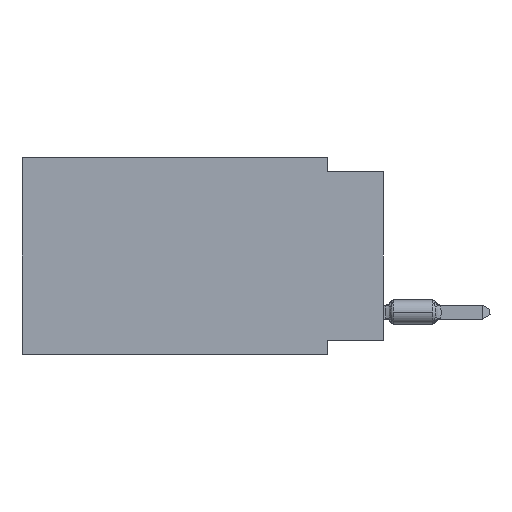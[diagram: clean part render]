
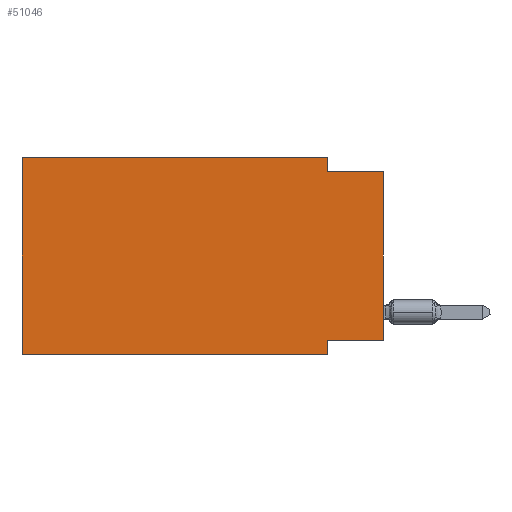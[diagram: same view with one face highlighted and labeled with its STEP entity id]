
A CAD part, left-side view. The second image highlights one B-rep face of the part: STEP entity #51046.
In plain terms, the highlighted planar face has unit normal (-1, 0, 0).
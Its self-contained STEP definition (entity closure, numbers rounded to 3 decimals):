
#1138 = ORIENTED_EDGE ( 'NONE', *, *, #31339, .F. ) ;
#1557 = VERTEX_POINT ( 'NONE', #15865 ) ;
#2071 = EDGE_CURVE ( 'NONE', #62082, #11415, #47600, .T. ) ;
#3947 = EDGE_CURVE ( 'NONE', #26505, #37810, #46423, .T. ) ;
#5848 = DIRECTION ( 'NONE',  ( 0., -1., 0. ) ) ;
#6095 = EDGE_CURVE ( 'NONE', #21302, #1557, #53220, .T. ) ;
#10886 = CARTESIAN_POINT ( 'NONE',  ( 0., 16.383, -8.89 ) ) ;
#10980 = CARTESIAN_POINT ( 'NONE',  ( 0., 16.383, 0. ) ) ;
#11415 = VERTEX_POINT ( 'NONE', #31381 ) ;
#11747 = CARTESIAN_POINT ( 'NONE',  ( 0., 0., -8.255 ) ) ;
#13044 = ORIENTED_EDGE ( 'NONE', *, *, #17821, .F. ) ;
#13174 = CARTESIAN_POINT ( 'NONE',  ( 0., 16.383, 0. ) ) ;
#14307 = ORIENTED_EDGE ( 'NONE', *, *, #48307, .T. ) ;
#15027 = CARTESIAN_POINT ( 'NONE',  ( 0., 2.54, -8.89 ) ) ;
#15865 = CARTESIAN_POINT ( 'NONE',  ( 0., 2.54, 0. ) ) ;
#16362 = PLANE ( 'NONE',  #42566 ) ;
#16434 = DIRECTION ( 'NONE',  ( 0., 1., 0. ) ) ;
#17821 = EDGE_CURVE ( 'NONE', #26505, #21302, #56416, .T. ) ;
#18202 = CARTESIAN_POINT ( 'NONE',  ( 0., 0., -8.255 ) ) ;
#19242 = LINE ( 'NONE', #28957, #56140 ) ;
#20790 = DIRECTION ( 'NONE',  ( 0., 0., 1. ) ) ;
#21302 = VERTEX_POINT ( 'NONE', #13174 ) ;
#22866 = VERTEX_POINT ( 'NONE', #36955 ) ;
#26079 = FACE_OUTER_BOUND ( 'NONE', #42232, .T. ) ;
#26472 = ORIENTED_EDGE ( 'NONE', *, *, #36853, .F. ) ;
#26487 = VECTOR ( 'NONE', #5848, 1000. ) ;
#26505 = VERTEX_POINT ( 'NONE', #48649 ) ;
#26892 = CARTESIAN_POINT ( 'NONE',  ( 0., 16.383, 0. ) ) ;
#28957 = CARTESIAN_POINT ( 'NONE',  ( 0., 0., -0.635 ) ) ;
#31339 = EDGE_CURVE ( 'NONE', #11415, #37810, #41487, .T. ) ;
#31381 = CARTESIAN_POINT ( 'NONE',  ( 0., 2.54, -8.255 ) ) ;
#31442 = DIRECTION ( 'NONE',  ( 0., 0., -1. ) ) ;
#31476 = ORIENTED_EDGE ( 'NONE', *, *, #64997, .F. ) ;
#31584 = DIRECTION ( 'NONE',  ( 0., 0., 1. ) ) ;
#31943 = VECTOR ( 'NONE', #20790, 1000. ) ;
#32130 = CARTESIAN_POINT ( 'NONE',  ( 0., 16.383, 0. ) ) ;
#36804 = DIRECTION ( 'NONE',  ( 1., 0., 0. ) ) ;
#36853 = EDGE_CURVE ( 'NONE', #1557, #38967, #57095, .T. ) ;
#36882 = VECTOR ( 'NONE', #31442, 1000. ) ;
#36955 = CARTESIAN_POINT ( 'NONE',  ( 0., 0., -0.635 ) ) ;
#37810 = VERTEX_POINT ( 'NONE', #57952 ) ;
#38967 = VERTEX_POINT ( 'NONE', #56730 ) ;
#41080 = ORIENTED_EDGE ( 'NONE', *, *, #3947, .T. ) ;
#41487 = LINE ( 'NONE', #15027, #36882 ) ;
#42232 = EDGE_LOOP ( 'NONE', ( #14307, #31476, #26472, #47606, #13044, #41080, #1138, #56118 ) ) ;
#42566 = AXIS2_PLACEMENT_3D ( 'NONE', #32130, #36804, #56618 ) ;
#46423 = LINE ( 'NONE', #10886, #26487 ) ;
#47600 = LINE ( 'NONE', #11747, #57360 ) ;
#47606 = ORIENTED_EDGE ( 'NONE', *, *, #6095, .F. ) ;
#48307 = EDGE_CURVE ( 'NONE', #62082, #22866, #61364, .T. ) ;
#48649 = CARTESIAN_POINT ( 'NONE',  ( 0., 16.383, -8.89 ) ) ;
#48747 = VECTOR ( 'NONE', #31584, 1000. ) ;
#49399 = DIRECTION ( 'NONE',  ( 0., -1., 0. ) ) ;
#51046 = ADVANCED_FACE ( 'NONE', ( #26079 ), #16362, .F. ) ;
#51198 = VECTOR ( 'NONE', #52722, 1000. ) ;
#52722 = DIRECTION ( 'NONE',  ( 0., 0., -1. ) ) ;
#53220 = LINE ( 'NONE', #10980, #55589 ) ;
#55589 = VECTOR ( 'NONE', #57613, 1000. ) ;
#56118 = ORIENTED_EDGE ( 'NONE', *, *, #2071, .F. ) ;
#56140 = VECTOR ( 'NONE', #49399, 1000. ) ;
#56336 = CARTESIAN_POINT ( 'NONE',  ( 0., 0., 0. ) ) ;
#56416 = LINE ( 'NONE', #26892, #48747 ) ;
#56618 = DIRECTION ( 'NONE',  ( 0., 0., -1. ) ) ;
#56730 = CARTESIAN_POINT ( 'NONE',  ( 0., 2.54, -0.635 ) ) ;
#57095 = LINE ( 'NONE', #57784, #51198 ) ;
#57360 = VECTOR ( 'NONE', #16434, 1000. ) ;
#57613 = DIRECTION ( 'NONE',  ( 0., -1., 0. ) ) ;
#57784 = CARTESIAN_POINT ( 'NONE',  ( 0., 2.54, 0. ) ) ;
#57952 = CARTESIAN_POINT ( 'NONE',  ( 0., 2.54, -8.89 ) ) ;
#61364 = LINE ( 'NONE', #56336, #31943 ) ;
#62082 = VERTEX_POINT ( 'NONE', #18202 ) ;
#64997 = EDGE_CURVE ( 'NONE', #38967, #22866, #19242, .T. ) ;
